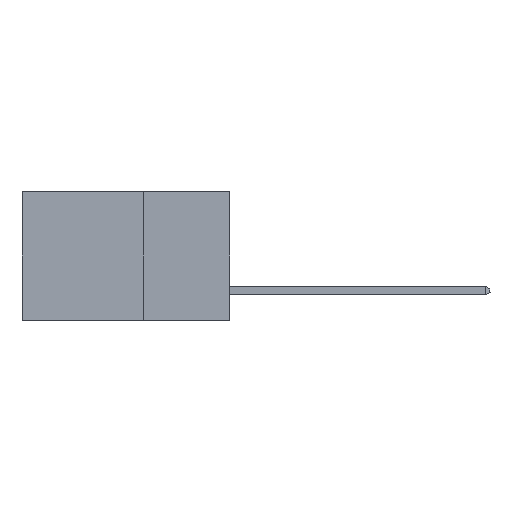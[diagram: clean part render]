
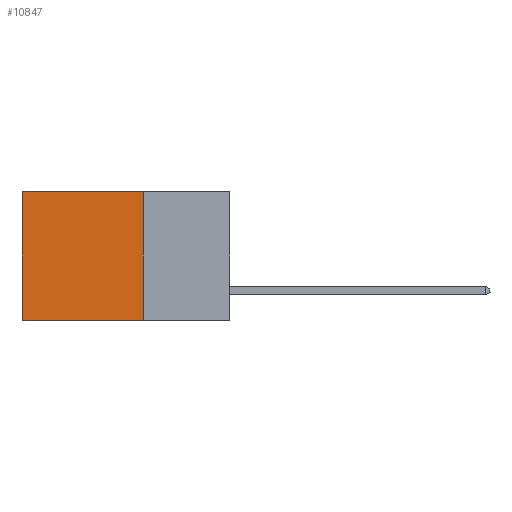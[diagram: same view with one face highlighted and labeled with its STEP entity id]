
A CAD part, left-side view. The second image highlights one B-rep face of the part: STEP entity #10847.
In plain terms, the highlighted planar face has unit normal (-1, 0, 0).
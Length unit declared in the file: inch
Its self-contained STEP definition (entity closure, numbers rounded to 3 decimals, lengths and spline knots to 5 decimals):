
#1003 = CARTESIAN_POINT ( 'NONE',  ( 0.298, 0.25, 0. ) ) ;
#1103 = EDGE_CURVE ( 'NONE', #7981, #9996, #13456, .T. ) ;
#2341 = AXIS2_PLACEMENT_3D ( 'NONE', #11269, #16768, #12862 ) ;
#2385 = LINE ( 'NONE', #13499, #16439 ) ;
#2390 = VERTEX_POINT ( 'NONE', #9893 ) ;
#4903 = EDGE_LOOP ( 'NONE', ( #8852, #5166, #17152, #13824 ) ) ;
#4921 = VECTOR ( 'NONE', #5667, 39.37008 ) ;
#5166 = ORIENTED_EDGE ( 'NONE', *, *, #11331, .F. ) ;
#5667 = DIRECTION ( 'NONE',  ( 0., 1., 0. ) ) ;
#6017 = PLANE ( 'NONE',  #2341 ) ;
#6429 = VECTOR ( 'NONE', #12379, 39.37008 ) ;
#7648 = CARTESIAN_POINT ( 'NONE',  ( 0.298, 0.6, 0. ) ) ;
#7981 = VERTEX_POINT ( 'NONE', #1003 ) ;
#8831 = EDGE_CURVE ( 'NONE', #10977, #2390, #8988, .T. ) ;
#8852 = ORIENTED_EDGE ( 'NONE', *, *, #8831, .T. ) ;
#8988 = LINE ( 'NONE', #16641, #6429 ) ;
#9343 = CARTESIAN_POINT ( 'NONE',  ( 0.298, 0.25, 0. ) ) ;
#9403 = DIRECTION ( 'NONE',  ( 0., 0., -1. ) ) ;
#9893 = CARTESIAN_POINT ( 'NONE',  ( 0.298, 0.6, -0.37 ) ) ;
#9996 = VERTEX_POINT ( 'NONE', #13254 ) ;
#10847 = ADVANCED_FACE ( 'NONE', ( #12124 ), #6017, .F. ) ;
#10977 = VERTEX_POINT ( 'NONE', #7648 ) ;
#11269 = CARTESIAN_POINT ( 'NONE',  ( 0.298, 0.25, 0. ) ) ;
#11331 = EDGE_CURVE ( 'NONE', #9996, #2390, #14906, .T. ) ;
#12124 = FACE_OUTER_BOUND ( 'NONE', #4903, .T. ) ;
#12379 = DIRECTION ( 'NONE',  ( 0., 0., -1. ) ) ;
#12497 = CARTESIAN_POINT ( 'NONE',  ( 0.298, 0.25, -0.37 ) ) ;
#12862 = DIRECTION ( 'NONE',  ( 0., 0., -1. ) ) ;
#13254 = CARTESIAN_POINT ( 'NONE',  ( 0.298, 0.25, -0.37 ) ) ;
#13456 = LINE ( 'NONE', #9343, #14732 ) ;
#13499 = CARTESIAN_POINT ( 'NONE',  ( 0.298, 0.25, 0. ) ) ;
#13824 = ORIENTED_EDGE ( 'NONE', *, *, #14140, .T. ) ;
#14140 = EDGE_CURVE ( 'NONE', #7981, #10977, #2385, .T. ) ;
#14732 = VECTOR ( 'NONE', #9403, 39.37008 ) ;
#14906 = LINE ( 'NONE', #12497, #4921 ) ;
#15024 = DIRECTION ( 'NONE',  ( 0., 1., 0. ) ) ;
#16439 = VECTOR ( 'NONE', #15024, 39.37008 ) ;
#16641 = CARTESIAN_POINT ( 'NONE',  ( 0.298, 0.6, 0. ) ) ;
#16768 = DIRECTION ( 'NONE',  ( 1., 0., 0. ) ) ;
#17152 = ORIENTED_EDGE ( 'NONE', *, *, #1103, .F. ) ;
